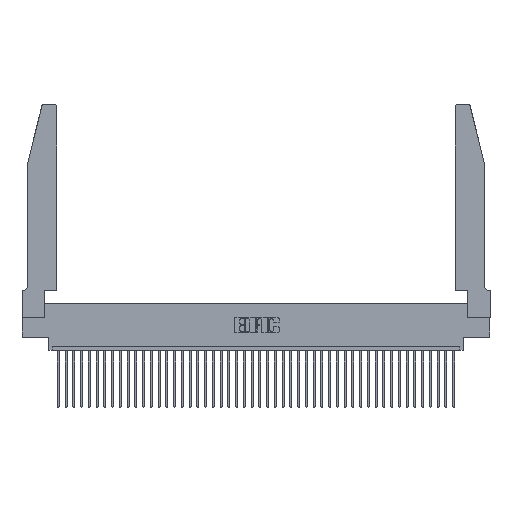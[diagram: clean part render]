
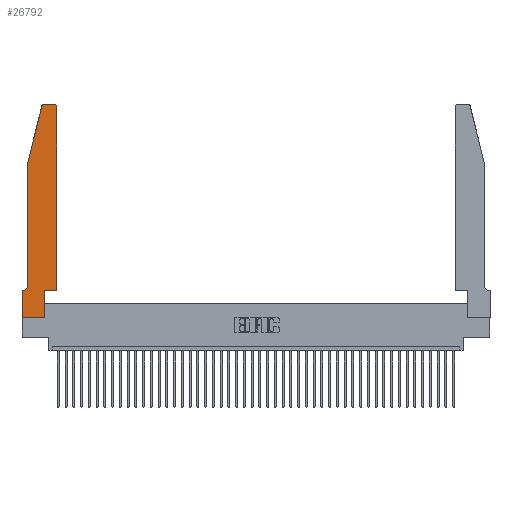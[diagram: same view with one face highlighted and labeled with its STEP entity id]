
A CAD part, top view. The second image highlights one B-rep face of the part: STEP entity #26792.
In plain terms, the highlighted planar face has unit normal (0, 0, 1).
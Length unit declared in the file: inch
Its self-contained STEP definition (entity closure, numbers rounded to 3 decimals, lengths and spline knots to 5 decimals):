
#557 = CARTESIAN_POINT ( 'NONE',  ( 0.2865, 0.35, 0.37 ) ) ;
#1021 = LINE ( 'NONE', #10759, #35470 ) ;
#1064 = DIRECTION ( 'NONE',  ( 0., 0., 1. ) ) ;
#1285 = DIRECTION ( 'NONE',  ( 1., 0., 0. ) ) ;
#2267 = CARTESIAN_POINT ( 'NONE',  ( 0.284, 2.75, 0.37 ) ) ;
#2326 = VECTOR ( 'NONE', #11168, 39.37008 ) ;
#2436 = CARTESIAN_POINT ( 'NONE',  ( 0.0755, 2., 0.37 ) ) ;
#3375 = CARTESIAN_POINT ( 'NONE',  ( 0.2865, 0., 0.37 ) ) ;
#4012 = EDGE_CURVE ( 'NONE', #4632, #19895, #41622, .T. ) ;
#4259 = LINE ( 'NONE', #27286, #28264 ) ;
#4632 = VERTEX_POINT ( 'NONE', #2436 ) ;
#4871 = CARTESIAN_POINT ( 'NONE',  ( 0., 0.35, 0.37 ) ) ;
#4990 = CARTESIAN_POINT ( 'NONE',  ( 0.0055, 0.42, 0.37 ) ) ;
#5585 = PLANE ( 'NONE',  #18819 ) ;
#5672 = DIRECTION ( 'NONE',  ( 1., 0., 0. ) ) ;
#6004 = CARTESIAN_POINT ( 'NONE',  ( 0., 0.35, 0.37 ) ) ;
#6028 = DIRECTION ( 'NONE',  ( 0., -1., 0. ) ) ;
#6150 = CARTESIAN_POINT ( 'NONE',  ( 0.0755, 0.35, 0.37 ) ) ;
#6299 = LINE ( 'NONE', #36912, #17028 ) ;
#6417 = CIRCLE ( 'NONE', #35538, 0.07 ) ;
#6639 = VECTOR ( 'NONE', #6028, 39.37008 ) ;
#7246 = EDGE_CURVE ( 'NONE', #37938, #11951, #24296, .T. ) ;
#7329 = ORIENTED_EDGE ( 'NONE', *, *, #8831, .T. ) ;
#7497 = EDGE_CURVE ( 'NONE', #11951, #13046, #6299, .T. ) ;
#7720 = DIRECTION ( 'NONE',  ( 1., 0., 0. ) ) ;
#7978 = LINE ( 'NONE', #30571, #2326 ) ;
#8168 = LINE ( 'NONE', #25710, #6639 ) ;
#8831 = EDGE_CURVE ( 'NONE', #19959, #16400, #8168, .T. ) ;
#9050 = ORIENTED_EDGE ( 'NONE', *, *, #21951, .T. ) ;
#10003 = ORIENTED_EDGE ( 'NONE', *, *, #24554, .T. ) ;
#10759 = CARTESIAN_POINT ( 'NONE',  ( 0.2605, 2.75, 0.37 ) ) ;
#11168 = DIRECTION ( 'NONE',  ( -0.239, -0.971, 0. ) ) ;
#11260 = CARTESIAN_POINT ( 'NONE',  ( 0.284, 2.72, 0.37 ) ) ;
#11951 = VERTEX_POINT ( 'NONE', #557 ) ;
#12105 = EDGE_CURVE ( 'NONE', #18101, #4632, #7978, .T. ) ;
#12835 = CARTESIAN_POINT ( 'NONE',  ( 0.25487, 2.72718, 0.37 ) ) ;
#12857 = ORIENTED_EDGE ( 'NONE', *, *, #40725, .T. ) ;
#13046 = VERTEX_POINT ( 'NONE', #40305 ) ;
#13268 = CIRCLE ( 'NONE', #38978, 0.03 ) ;
#14570 = DIRECTION ( 'NONE',  ( 0., 0., -1. ) ) ;
#15254 = CARTESIAN_POINT ( 'NONE',  ( 0., 0., 0.37 ) ) ;
#15861 = DIRECTION ( 'NONE',  ( -1., 0., 0. ) ) ;
#16207 = AXIS2_PLACEMENT_3D ( 'NONE', #11260, #1064, #24067 ) ;
#16400 = VERTEX_POINT ( 'NONE', #15254 ) ;
#17028 = VECTOR ( 'NONE', #7720, 39.37008 ) ;
#17862 = CARTESIAN_POINT ( 'NONE',  ( 0.4205, 2.72, 0.37 ) ) ;
#18101 = VERTEX_POINT ( 'NONE', #12835 ) ;
#18741 = ORIENTED_EDGE ( 'NONE', *, *, #25627, .T. ) ;
#18819 = AXIS2_PLACEMENT_3D ( 'NONE', #6004, #22076, #28969 ) ;
#19895 = VERTEX_POINT ( 'NONE', #42162 ) ;
#19959 = VERTEX_POINT ( 'NONE', #4871 ) ;
#20526 = CIRCLE ( 'NONE', #16207, 0.03 ) ;
#20756 = VERTEX_POINT ( 'NONE', #25892 ) ;
#21015 = EDGE_CURVE ( 'NONE', #25618, #33159, #1021, .T. ) ;
#21149 = DIRECTION ( 'NONE',  ( 0., 0., 1. ) ) ;
#21499 = CARTESIAN_POINT ( 'NONE',  ( 0.0755, 2., 0.37 ) ) ;
#21951 = EDGE_CURVE ( 'NONE', #19895, #20756, #6417, .T. ) ;
#22076 = DIRECTION ( 'NONE',  ( 0., 0., 1. ) ) ;
#23982 = DIRECTION ( 'NONE',  ( -1., 0., 0. ) ) ;
#24067 = DIRECTION ( 'NONE',  ( 1., 0., 0. ) ) ;
#24296 = LINE ( 'NONE', #28312, #32012 ) ;
#24483 = ORIENTED_EDGE ( 'NONE', *, *, #32979, .T. ) ;
#24534 = ORIENTED_EDGE ( 'NONE', *, *, #25848, .T. ) ;
#24554 = EDGE_CURVE ( 'NONE', #13046, #36256, #33387, .T. ) ;
#25618 = VERTEX_POINT ( 'NONE', #29249 ) ;
#25627 = EDGE_CURVE ( 'NONE', #20756, #19959, #28243, .T. ) ;
#25710 = CARTESIAN_POINT ( 'NONE',  ( 0., 0., 0.37 ) ) ;
#25848 = EDGE_CURVE ( 'NONE', #36256, #25618, #13268, .T. ) ;
#25892 = CARTESIAN_POINT ( 'NONE',  ( 0.0055, 0.35, 0.37 ) ) ;
#26598 = FACE_OUTER_BOUND ( 'NONE', #32645, .T. ) ;
#26792 = ADVANCED_FACE ( 'NONE', ( #26598 ), #5585, .T. ) ;
#27286 = CARTESIAN_POINT ( 'NONE',  ( 0., 0., 0.37 ) ) ;
#27835 = DIRECTION ( 'NONE',  ( -1., 0., 0. ) ) ;
#28243 = LINE ( 'NONE', #6150, #34884 ) ;
#28264 = VECTOR ( 'NONE', #1285, 39.37008 ) ;
#28312 = CARTESIAN_POINT ( 'NONE',  ( 0.2865, 0.35, 0.37 ) ) ;
#28969 = DIRECTION ( 'NONE',  ( 1., 0., 0. ) ) ;
#29249 = CARTESIAN_POINT ( 'NONE',  ( 0.4205, 2.75, 0.37 ) ) ;
#30571 = CARTESIAN_POINT ( 'NONE',  ( 0.0755, 2., 0.37 ) ) ;
#30670 = VECTOR ( 'NONE', #38651, 39.37008 ) ;
#31816 = CARTESIAN_POINT ( 'NONE',  ( 0.4505, 0.35, 0.37 ) ) ;
#32012 = VECTOR ( 'NONE', #35363, 39.37008 ) ;
#32645 = EDGE_LOOP ( 'NONE', ( #40652, #12857, #37559, #41216, #9050, #18741, #7329, #24483, #42297, #34874, #10003, #24534 ) ) ;
#32979 = EDGE_CURVE ( 'NONE', #16400, #37938, #4259, .T. ) ;
#33159 = VERTEX_POINT ( 'NONE', #2267 ) ;
#33387 = LINE ( 'NONE', #31816, #39635 ) ;
#33762 = CARTESIAN_POINT ( 'NONE',  ( 0.4505, 2.72, 0.37 ) ) ;
#34874 = ORIENTED_EDGE ( 'NONE', *, *, #7497, .T. ) ;
#34884 = VECTOR ( 'NONE', #15861, 39.37008 ) ;
#35363 = DIRECTION ( 'NONE',  ( 0., 1., 0. ) ) ;
#35470 = VECTOR ( 'NONE', #23982, 39.37008 ) ;
#35538 = AXIS2_PLACEMENT_3D ( 'NONE', #4990, #14570, #27835 ) ;
#36256 = VERTEX_POINT ( 'NONE', #33762 ) ;
#36912 = CARTESIAN_POINT ( 'NONE',  ( 0.4505, 0.35, 0.37 ) ) ;
#37559 = ORIENTED_EDGE ( 'NONE', *, *, #12105, .T. ) ;
#37938 = VERTEX_POINT ( 'NONE', #3375 ) ;
#38651 = DIRECTION ( 'NONE',  ( 0., -1., 0. ) ) ;
#38978 = AXIS2_PLACEMENT_3D ( 'NONE', #17862, #21149, #5672 ) ;
#39635 = VECTOR ( 'NONE', #41723, 39.37008 ) ;
#40305 = CARTESIAN_POINT ( 'NONE',  ( 0.4505, 0.35, 0.37 ) ) ;
#40652 = ORIENTED_EDGE ( 'NONE', *, *, #21015, .T. ) ;
#40725 = EDGE_CURVE ( 'NONE', #33159, #18101, #20526, .T. ) ;
#41216 = ORIENTED_EDGE ( 'NONE', *, *, #4012, .T. ) ;
#41622 = LINE ( 'NONE', #21499, #30670 ) ;
#41723 = DIRECTION ( 'NONE',  ( 0., 1., 0. ) ) ;
#42162 = CARTESIAN_POINT ( 'NONE',  ( 0.0755, 0.42, 0.37 ) ) ;
#42297 = ORIENTED_EDGE ( 'NONE', *, *, #7246, .T. ) ;
